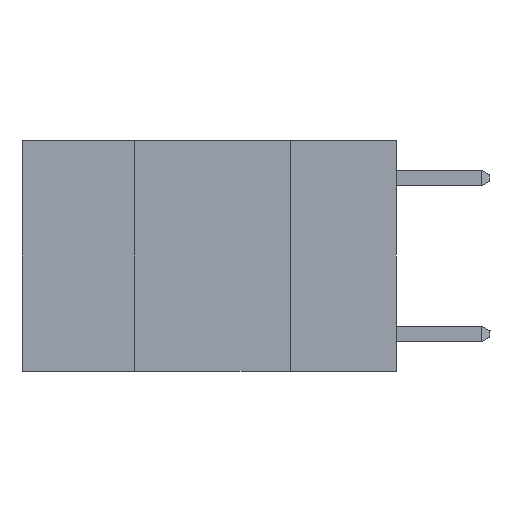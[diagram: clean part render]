
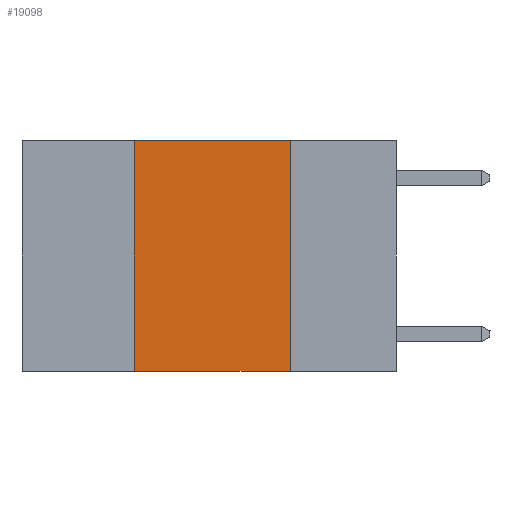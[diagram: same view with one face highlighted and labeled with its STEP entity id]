
A CAD part, left-side view. The second image highlights one B-rep face of the part: STEP entity #19098.
In plain terms, the highlighted planar face has unit normal (-1, 0, 0).
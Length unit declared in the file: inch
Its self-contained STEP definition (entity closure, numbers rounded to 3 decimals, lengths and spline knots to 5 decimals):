
#781 = DIRECTION ( 'NONE',  ( 0., 0., -1. ) ) ;
#1030 = CARTESIAN_POINT ( 'NONE',  ( 0., 0.42, 0. ) ) ;
#1341 = VERTEX_POINT ( 'NONE', #4952 ) ;
#1976 = PLANE ( 'NONE',  #16817 ) ;
#2558 = DIRECTION ( 'NONE',  ( 0., 0., 1. ) ) ;
#3491 = DIRECTION ( 'NONE',  ( 1., 0., 0. ) ) ;
#3865 = CARTESIAN_POINT ( 'NONE',  ( 0., 0.42, -0.37 ) ) ;
#4786 = VERTEX_POINT ( 'NONE', #15784 ) ;
#4952 = CARTESIAN_POINT ( 'NONE',  ( 0., 0.17, -0.37 ) ) ;
#5054 = LINE ( 'NONE', #7750, #13160 ) ;
#6242 = VECTOR ( 'NONE', #2558, 39.37008 ) ;
#6517 = VERTEX_POINT ( 'NONE', #15415 ) ;
#6815 = VECTOR ( 'NONE', #15799, 39.37008 ) ;
#7750 = CARTESIAN_POINT ( 'NONE',  ( 0., 0.6, -0.37 ) ) ;
#9829 = CARTESIAN_POINT ( 'NONE',  ( 0., 0.6, 0. ) ) ;
#10660 = VECTOR ( 'NONE', #781, 39.37008 ) ;
#11963 = EDGE_CURVE ( 'NONE', #6517, #4786, #19154, .T. ) ;
#12007 = ORIENTED_EDGE ( 'NONE', *, *, #14878, .F. ) ;
#12630 = CARTESIAN_POINT ( 'NONE',  ( 0., 0.6, 0. ) ) ;
#12996 = CARTESIAN_POINT ( 'NONE',  ( 0., 0.17, 0. ) ) ;
#13160 = VECTOR ( 'NONE', #18151, 39.37008 ) ;
#13257 = ORIENTED_EDGE ( 'NONE', *, *, #17732, .T. ) ;
#13377 = FACE_OUTER_BOUND ( 'NONE', #18257, .T. ) ;
#14102 = ORIENTED_EDGE ( 'NONE', *, *, #11963, .F. ) ;
#14132 = DIRECTION ( 'NONE',  ( 0., 0., -1. ) ) ;
#14878 = EDGE_CURVE ( 'NONE', #4786, #1341, #18485, .T. ) ;
#15126 = ORIENTED_EDGE ( 'NONE', *, *, #16811, .F. ) ;
#15415 = CARTESIAN_POINT ( 'NONE',  ( 0., 0.42, 0. ) ) ;
#15784 = CARTESIAN_POINT ( 'NONE',  ( 0., 0.17, 0. ) ) ;
#15799 = DIRECTION ( 'NONE',  ( 0., -1., 0. ) ) ;
#16811 = EDGE_CURVE ( 'NONE', #18048, #6517, #18171, .T. ) ;
#16817 = AXIS2_PLACEMENT_3D ( 'NONE', #12630, #3491, #14132 ) ;
#17732 = EDGE_CURVE ( 'NONE', #18048, #1341, #5054, .T. ) ;
#18048 = VERTEX_POINT ( 'NONE', #3865 ) ;
#18151 = DIRECTION ( 'NONE',  ( 0., -1., 0. ) ) ;
#18171 = LINE ( 'NONE', #1030, #6242 ) ;
#18257 = EDGE_LOOP ( 'NONE', ( #12007, #14102, #15126, #13257 ) ) ;
#18485 = LINE ( 'NONE', #12996, #10660 ) ;
#19098 = ADVANCED_FACE ( 'NONE', ( #13377 ), #1976, .F. ) ;
#19154 = LINE ( 'NONE', #9829, #6815 ) ;
